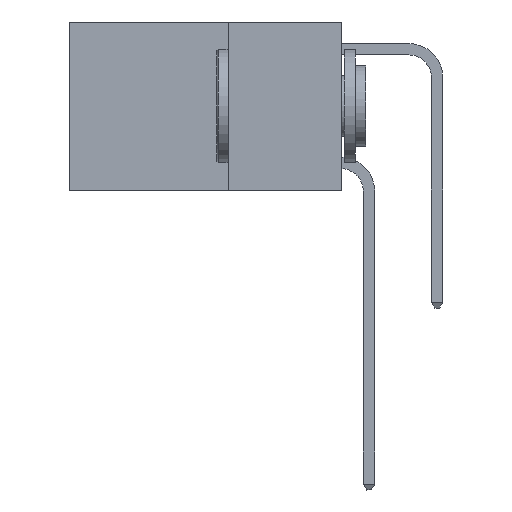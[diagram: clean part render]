
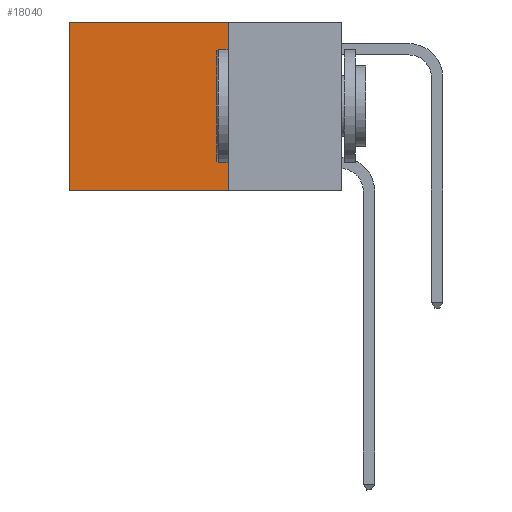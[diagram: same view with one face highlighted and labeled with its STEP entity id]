
A CAD part, left-side view. The second image highlights one B-rep face of the part: STEP entity #18040.
In plain terms, the highlighted planar face has unit normal (-1, 0, 0).
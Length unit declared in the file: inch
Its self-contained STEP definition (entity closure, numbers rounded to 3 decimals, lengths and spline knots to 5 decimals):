
#117 = VECTOR ( 'NONE', #452, 39.37008 ) ;
#452 = DIRECTION ( 'NONE',  ( 0., 1., 0. ) ) ;
#1644 = DIRECTION ( 'NONE',  ( 1., 0., 0. ) ) ;
#1789 = CARTESIAN_POINT ( 'NONE',  ( 0.2625, 0.25, 0. ) ) ;
#2095 = EDGE_LOOP ( 'NONE', ( #15071, #15036, #18809, #3445 ) ) ;
#2897 = VECTOR ( 'NONE', #8512, 39.37008 ) ;
#3216 = VERTEX_POINT ( 'NONE', #12844 ) ;
#3445 = ORIENTED_EDGE ( 'NONE', *, *, #7683, .T. ) ;
#3828 = FACE_OUTER_BOUND ( 'NONE', #2095, .T. ) ;
#4245 = EDGE_CURVE ( 'NONE', #12767, #4662, #15700, .T. ) ;
#4501 = VERTEX_POINT ( 'NONE', #7772 ) ;
#4662 = VERTEX_POINT ( 'NONE', #9776 ) ;
#4929 = VECTOR ( 'NONE', #11116, 39.37008 ) ;
#5497 = CARTESIAN_POINT ( 'NONE',  ( 0.2625, 0.25, -0.37 ) ) ;
#7683 = EDGE_CURVE ( 'NONE', #3216, #4501, #9176, .T. ) ;
#7772 = CARTESIAN_POINT ( 'NONE',  ( 0.2625, 0.6, 0. ) ) ;
#7927 = EDGE_CURVE ( 'NONE', #4501, #4662, #13291, .T. ) ;
#8039 = AXIS2_PLACEMENT_3D ( 'NONE', #11711, #1644, #13360 ) ;
#8359 = PLANE ( 'NONE',  #8039 ) ;
#8512 = DIRECTION ( 'NONE',  ( 0., 0., -1. ) ) ;
#9176 = LINE ( 'NONE', #20463, #117 ) ;
#9776 = CARTESIAN_POINT ( 'NONE',  ( 0.2625, 0.6, -0.37 ) ) ;
#11116 = DIRECTION ( 'NONE',  ( 0., 0., -1. ) ) ;
#11711 = CARTESIAN_POINT ( 'NONE',  ( 0.2625, 0.25, 0. ) ) ;
#12401 = EDGE_CURVE ( 'NONE', #3216, #12767, #20078, .T. ) ;
#12767 = VERTEX_POINT ( 'NONE', #19256 ) ;
#12844 = CARTESIAN_POINT ( 'NONE',  ( 0.2625, 0.25, 0. ) ) ;
#13291 = LINE ( 'NONE', #20943, #4929 ) ;
#13360 = DIRECTION ( 'NONE',  ( 0., 0., -1. ) ) ;
#15036 = ORIENTED_EDGE ( 'NONE', *, *, #4245, .F. ) ;
#15071 = ORIENTED_EDGE ( 'NONE', *, *, #7927, .T. ) ;
#15700 = LINE ( 'NONE', #5497, #17308 ) ;
#17308 = VECTOR ( 'NONE', #18800, 39.37008 ) ;
#18040 = ADVANCED_FACE ( 'NONE', ( #3828 ), #8359, .F. ) ;
#18800 = DIRECTION ( 'NONE',  ( 0., 1., 0. ) ) ;
#18809 = ORIENTED_EDGE ( 'NONE', *, *, #12401, .F. ) ;
#19256 = CARTESIAN_POINT ( 'NONE',  ( 0.2625, 0.25, -0.37 ) ) ;
#20078 = LINE ( 'NONE', #1789, #2897 ) ;
#20463 = CARTESIAN_POINT ( 'NONE',  ( 0.2625, 0.25, 0. ) ) ;
#20943 = CARTESIAN_POINT ( 'NONE',  ( 0.2625, 0.6, 0. ) ) ;
